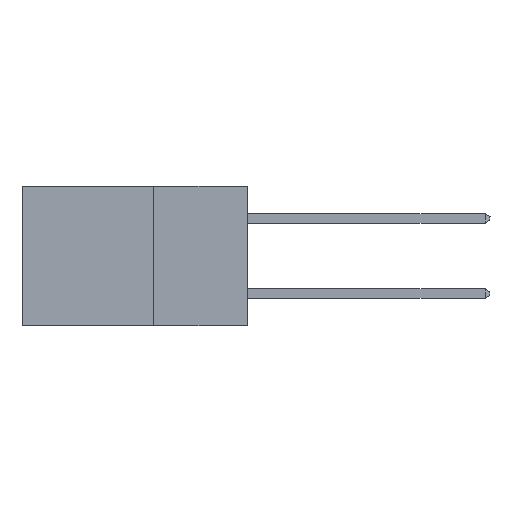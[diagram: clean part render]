
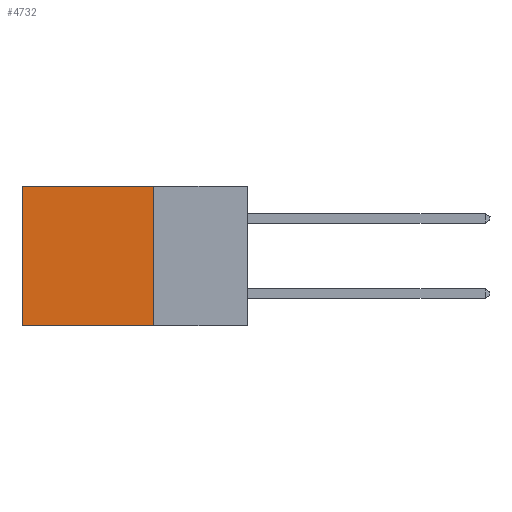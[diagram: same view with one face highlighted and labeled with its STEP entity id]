
A CAD part, left-side view. The second image highlights one B-rep face of the part: STEP entity #4732.
In plain terms, the highlighted planar face has unit normal (-1, 0, 0).
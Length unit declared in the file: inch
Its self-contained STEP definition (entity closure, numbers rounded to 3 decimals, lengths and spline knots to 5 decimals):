
#401 = VERTEX_POINT ( 'NONE', #6490 ) ;
#715 = LINE ( 'NONE', #9984, #5120 ) ;
#1065 = DIRECTION ( 'NONE',  ( 0., 1., 0. ) ) ;
#1430 = ORIENTED_EDGE ( 'NONE', *, *, #13458, .T. ) ;
#1965 = EDGE_CURVE ( 'NONE', #401, #12160, #5147, .T. ) ;
#2682 = CARTESIAN_POINT ( 'NONE',  ( 0.2615, 0.6, 0. ) ) ;
#2689 = EDGE_CURVE ( 'NONE', #401, #3661, #5340, .T. ) ;
#3455 = VERTEX_POINT ( 'NONE', #10813 ) ;
#3661 = VERTEX_POINT ( 'NONE', #6960 ) ;
#4732 = ADVANCED_FACE ( 'NONE', ( #12637 ), #11723, .F. ) ;
#5120 = VECTOR ( 'NONE', #11439, 39.37008 ) ;
#5147 = LINE ( 'NONE', #8432, #5245 ) ;
#5245 = VECTOR ( 'NONE', #1065, 39.37008 ) ;
#5291 = DIRECTION ( 'NONE',  ( 1., 0., 0. ) ) ;
#5340 = LINE ( 'NONE', #11054, #7518 ) ;
#5595 = ORIENTED_EDGE ( 'NONE', *, *, #2689, .F. ) ;
#6490 = CARTESIAN_POINT ( 'NONE',  ( 0.2615, 0.25, 0. ) ) ;
#6661 = VECTOR ( 'NONE', #11166, 39.37008 ) ;
#6900 = CARTESIAN_POINT ( 'NONE',  ( 0.2615, 0.25, -0.37 ) ) ;
#6960 = CARTESIAN_POINT ( 'NONE',  ( 0.2615, 0.25, -0.37 ) ) ;
#7064 = CARTESIAN_POINT ( 'NONE',  ( 0.2615, 0.25, -0.37 ) ) ;
#7518 = VECTOR ( 'NONE', #9593, 39.37008 ) ;
#8287 = LINE ( 'NONE', #6900, #6661 ) ;
#8432 = CARTESIAN_POINT ( 'NONE',  ( 0.2615, 0.25, 0. ) ) ;
#9593 = DIRECTION ( 'NONE',  ( 0., 0., -1. ) ) ;
#9984 = CARTESIAN_POINT ( 'NONE',  ( 0.2615, 0.6, -0.37 ) ) ;
#10272 = DIRECTION ( 'NONE',  ( 0., 0., -1. ) ) ;
#10813 = CARTESIAN_POINT ( 'NONE',  ( 0.2615, 0.6, -0.37 ) ) ;
#10917 = AXIS2_PLACEMENT_3D ( 'NONE', #7064, #5291, #10272 ) ;
#11054 = CARTESIAN_POINT ( 'NONE',  ( 0.2615, 0.25, -0.37 ) ) ;
#11166 = DIRECTION ( 'NONE',  ( 0., 1., 0. ) ) ;
#11439 = DIRECTION ( 'NONE',  ( 0., 0., -1. ) ) ;
#11723 = PLANE ( 'NONE',  #10917 ) ;
#11882 = EDGE_LOOP ( 'NONE', ( #1430, #12196, #5595, #12626 ) ) ;
#12073 = EDGE_CURVE ( 'NONE', #3661, #3455, #8287, .T. ) ;
#12160 = VERTEX_POINT ( 'NONE', #2682 ) ;
#12196 = ORIENTED_EDGE ( 'NONE', *, *, #12073, .F. ) ;
#12626 = ORIENTED_EDGE ( 'NONE', *, *, #1965, .T. ) ;
#12637 = FACE_OUTER_BOUND ( 'NONE', #11882, .T. ) ;
#13458 = EDGE_CURVE ( 'NONE', #12160, #3455, #715, .T. ) ;
